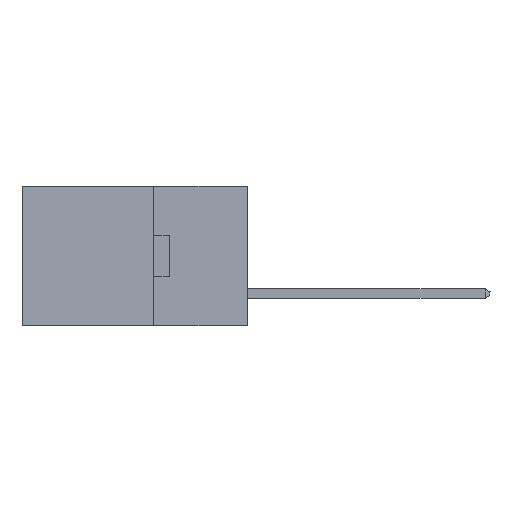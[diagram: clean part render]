
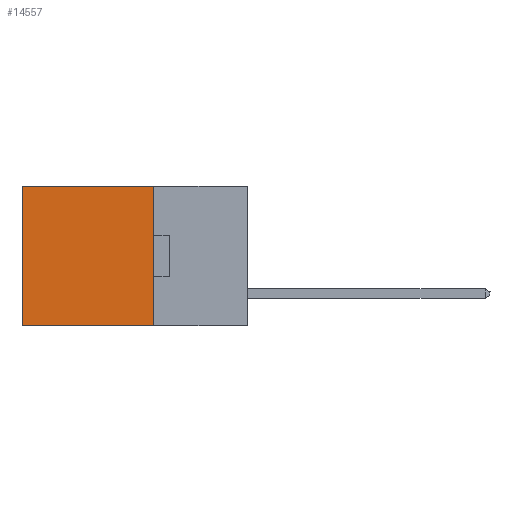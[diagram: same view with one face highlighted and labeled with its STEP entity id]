
A CAD part, left-side view. The second image highlights one B-rep face of the part: STEP entity #14557.
In plain terms, the highlighted planar face has unit normal (-1, 0, 0).
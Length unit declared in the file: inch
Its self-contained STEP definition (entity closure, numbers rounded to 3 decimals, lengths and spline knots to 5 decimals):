
#1174 = VERTEX_POINT ( 'NONE', #12104 ) ;
#1298 = VECTOR ( 'NONE', #19295, 39.37008 ) ;
#2739 = LINE ( 'NONE', #11151, #1298 ) ;
#2804 = ORIENTED_EDGE ( 'NONE', *, *, #6234, .T. ) ;
#3030 = LINE ( 'NONE', #22813, #17892 ) ;
#3465 = VERTEX_POINT ( 'NONE', #5787 ) ;
#3998 = PLANE ( 'NONE',  #9127 ) ;
#4127 = DIRECTION ( 'NONE',  ( 0., 0., -1. ) ) ;
#4635 = CARTESIAN_POINT ( 'NONE',  ( 0.2615, 0.25, 0. ) ) ;
#5119 = EDGE_CURVE ( 'NONE', #15984, #1174, #10201, .T. ) ;
#5493 = LINE ( 'NONE', #25659, #15746 ) ;
#5787 = CARTESIAN_POINT ( 'NONE',  ( 0.2615, 0.6, 0. ) ) ;
#6048 = EDGE_CURVE ( 'NONE', #3465, #17891, #3030, .T. ) ;
#6234 = EDGE_CURVE ( 'NONE', #15984, #3465, #5493, .T. ) ;
#7050 = ORIENTED_EDGE ( 'NONE', *, *, #5119, .F. ) ;
#8193 = DIRECTION ( 'NONE',  ( 0., 0., -1. ) ) ;
#9127 = AXIS2_PLACEMENT_3D ( 'NONE', #12140, #20284, #4127 ) ;
#9385 = ORIENTED_EDGE ( 'NONE', *, *, #17695, .F. ) ;
#10201 = LINE ( 'NONE', #18333, #11457 ) ;
#11151 = CARTESIAN_POINT ( 'NONE',  ( 0.2615, 0.25, -0.37 ) ) ;
#11182 = DIRECTION ( 'NONE',  ( 0., 0., -1. ) ) ;
#11457 = VECTOR ( 'NONE', #8193, 39.37008 ) ;
#11665 = CARTESIAN_POINT ( 'NONE',  ( 0.2615, 0.6, -0.37 ) ) ;
#12104 = CARTESIAN_POINT ( 'NONE',  ( 0.2615, 0.25, -0.37 ) ) ;
#12140 = CARTESIAN_POINT ( 'NONE',  ( 0.2615, 0.25, -0.37 ) ) ;
#13806 = EDGE_LOOP ( 'NONE', ( #15633, #9385, #7050, #2804 ) ) ;
#13861 = DIRECTION ( 'NONE',  ( 0., 1., 0. ) ) ;
#14557 = ADVANCED_FACE ( 'NONE', ( #26178 ), #3998, .F. ) ;
#15633 = ORIENTED_EDGE ( 'NONE', *, *, #6048, .T. ) ;
#15746 = VECTOR ( 'NONE', #13861, 39.37008 ) ;
#15984 = VERTEX_POINT ( 'NONE', #4635 ) ;
#17695 = EDGE_CURVE ( 'NONE', #1174, #17891, #2739, .T. ) ;
#17891 = VERTEX_POINT ( 'NONE', #11665 ) ;
#17892 = VECTOR ( 'NONE', #11182, 39.37008 ) ;
#18333 = CARTESIAN_POINT ( 'NONE',  ( 0.2615, 0.25, -0.37 ) ) ;
#19295 = DIRECTION ( 'NONE',  ( 0., 1., 0. ) ) ;
#20284 = DIRECTION ( 'NONE',  ( 1., 0., 0. ) ) ;
#22813 = CARTESIAN_POINT ( 'NONE',  ( 0.2615, 0.6, -0.37 ) ) ;
#25659 = CARTESIAN_POINT ( 'NONE',  ( 0.2615, 0.25, 0. ) ) ;
#26178 = FACE_OUTER_BOUND ( 'NONE', #13806, .T. ) ;
